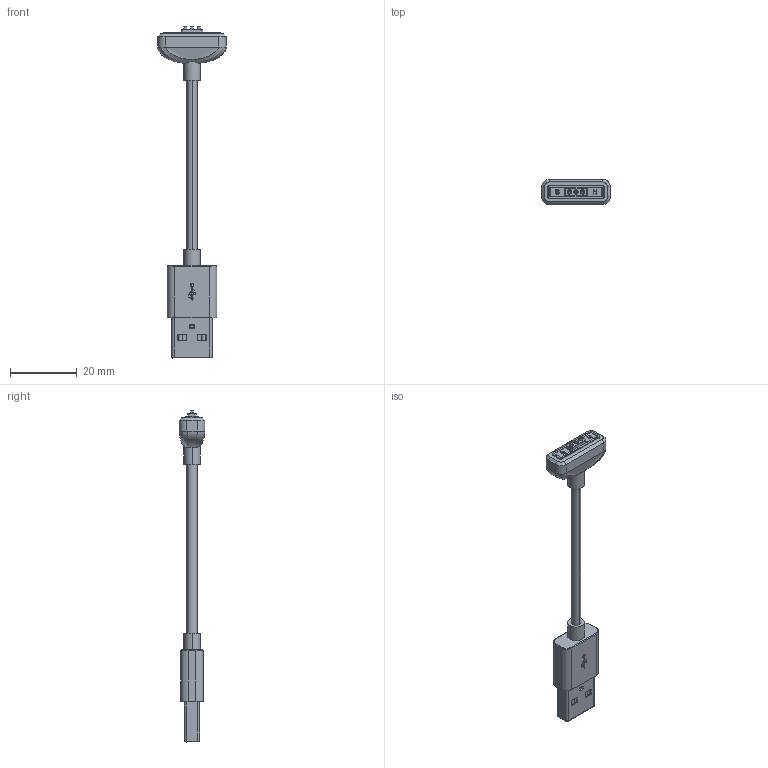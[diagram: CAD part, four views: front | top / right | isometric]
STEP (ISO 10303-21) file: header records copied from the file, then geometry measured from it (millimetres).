
FILE_DESCRIPTION (( 'STEP AP203' ), '1' );
FILE_NAME ('687-F0321A51110E.STEP', '2023-02-20T11:24:37', ( 'Magnum' ), ( '' ), 'SwSTEP 2.0', 'SolidWorks 2020', '' );
FILE_SCHEMA (( 'CONFIG_CONTROL_DESIGN' ));
Products named in the file (1): 687-F0321A51110E
Bounding box: 20.5 x 7.6 x 99.5 mm (x, y, z)
Volume: 3787 mm3; surface area: 5350.6 mm2
Topology: 8 solids, 9 shells, 1115 faces, 2961 edges, 1831 vertices
Faces by surface type: plane 580, cylinder 344, bspline 100, cone 43, torus 42, sphere 6
Entity records: 45917 total; most frequent: CARTESIAN_POINT 23832, ORIENTED_EDGE 5878, EDGE_CURVE 2939, B_SPLINE_CURVE_WITH_KNOTS 2557, DIRECTION 2487, VERTEX_POINT 1831, EDGE_LOOP 1188, AXIS2_PLACEMENT_3D 1126
